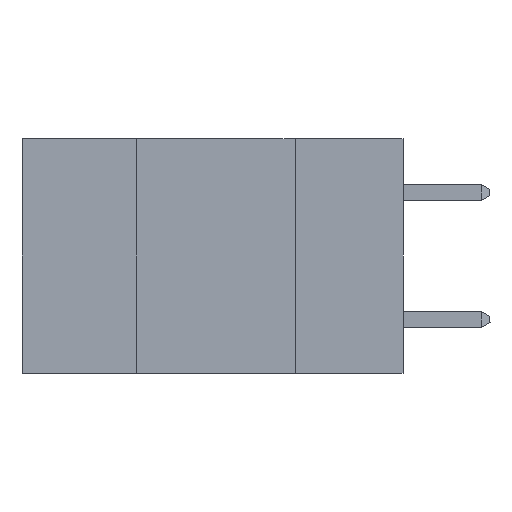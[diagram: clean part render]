
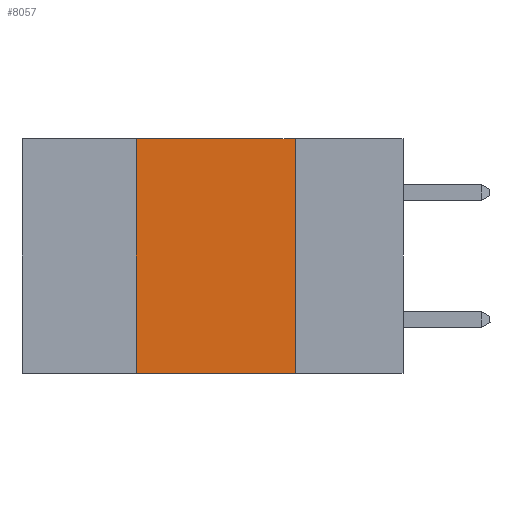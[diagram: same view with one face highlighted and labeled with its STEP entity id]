
A CAD part, left-side view. The second image highlights one B-rep face of the part: STEP entity #8057.
In plain terms, the highlighted planar face has unit normal (-1, 0, 0).
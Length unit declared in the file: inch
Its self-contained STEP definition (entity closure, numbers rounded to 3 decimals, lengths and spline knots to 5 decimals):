
#250 = LINE ( 'NONE', #16174, #15874 ) ;
#1882 = DIRECTION ( 'NONE',  ( 0., -1., 0. ) ) ;
#2518 = LINE ( 'NONE', #12202, #9112 ) ;
#3411 = VECTOR ( 'NONE', #8481, 39.37008 ) ;
#4458 = ORIENTED_EDGE ( 'NONE', *, *, #12322, .F. ) ;
#4587 = CARTESIAN_POINT ( 'NONE',  ( 0., 0.42, 0. ) ) ;
#5079 = EDGE_CURVE ( 'NONE', #14481, #17696, #250, .T. ) ;
#5406 = AXIS2_PLACEMENT_3D ( 'NONE', #7447, #15145, #19809 ) ;
#5456 = FACE_OUTER_BOUND ( 'NONE', #18610, .T. ) ;
#6039 = CARTESIAN_POINT ( 'NONE',  ( 0., 0.42, -0.37 ) ) ;
#7447 = CARTESIAN_POINT ( 'NONE',  ( 0., 0.6, 0. ) ) ;
#8022 = EDGE_CURVE ( 'NONE', #14481, #12702, #16392, .T. ) ;
#8057 = ADVANCED_FACE ( 'NONE', ( #5456 ), #11817, .F. ) ;
#8180 = CARTESIAN_POINT ( 'NONE',  ( 0., 0.42, 0. ) ) ;
#8181 = CARTESIAN_POINT ( 'NONE',  ( 0., 0.17, -0.37 ) ) ;
#8481 = DIRECTION ( 'NONE',  ( 0., 0., 1. ) ) ;
#8990 = ORIENTED_EDGE ( 'NONE', *, *, #5079, .T. ) ;
#9112 = VECTOR ( 'NONE', #10631, 39.37008 ) ;
#10020 = DIRECTION ( 'NONE',  ( 0., -1., 0. ) ) ;
#10450 = CARTESIAN_POINT ( 'NONE',  ( 0., 0.17, 0. ) ) ;
#10631 = DIRECTION ( 'NONE',  ( 0., 0., -1. ) ) ;
#11278 = CARTESIAN_POINT ( 'NONE',  ( 0., 0.6, 0. ) ) ;
#11817 = PLANE ( 'NONE',  #5406 ) ;
#12202 = CARTESIAN_POINT ( 'NONE',  ( 0., 0.17, 0. ) ) ;
#12322 = EDGE_CURVE ( 'NONE', #12702, #17773, #17910, .T. ) ;
#12492 = EDGE_CURVE ( 'NONE', #17773, #17696, #2518, .T. ) ;
#12588 = ORIENTED_EDGE ( 'NONE', *, *, #12492, .F. ) ;
#12702 = VERTEX_POINT ( 'NONE', #4587 ) ;
#14481 = VERTEX_POINT ( 'NONE', #6039 ) ;
#15145 = DIRECTION ( 'NONE',  ( 1., 0., 0. ) ) ;
#15874 = VECTOR ( 'NONE', #10020, 39.37008 ) ;
#16174 = CARTESIAN_POINT ( 'NONE',  ( 0., 0.6, -0.37 ) ) ;
#16392 = LINE ( 'NONE', #8180, #3411 ) ;
#17696 = VERTEX_POINT ( 'NONE', #8181 ) ;
#17773 = VERTEX_POINT ( 'NONE', #10450 ) ;
#17910 = LINE ( 'NONE', #11278, #20130 ) ;
#18610 = EDGE_LOOP ( 'NONE', ( #12588, #4458, #20219, #8990 ) ) ;
#19809 = DIRECTION ( 'NONE',  ( 0., 0., -1. ) ) ;
#20130 = VECTOR ( 'NONE', #1882, 39.37008 ) ;
#20219 = ORIENTED_EDGE ( 'NONE', *, *, #8022, .F. ) ;
